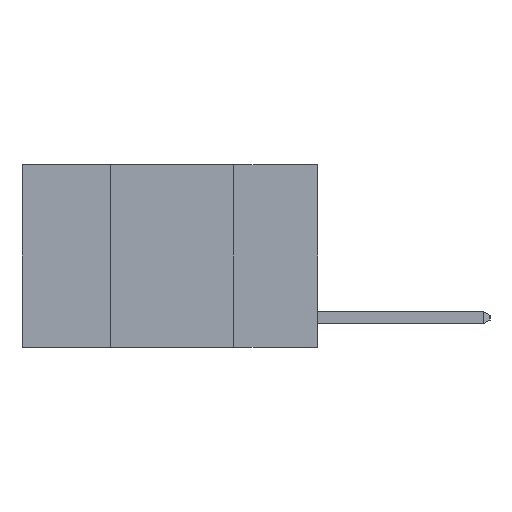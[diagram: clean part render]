
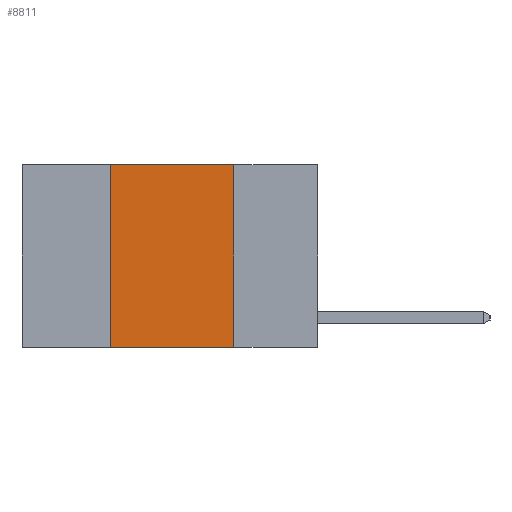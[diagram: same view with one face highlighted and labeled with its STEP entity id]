
A CAD part, left-side view. The second image highlights one B-rep face of the part: STEP entity #8811.
In plain terms, the highlighted planar face has unit normal (-1, 0, 0).
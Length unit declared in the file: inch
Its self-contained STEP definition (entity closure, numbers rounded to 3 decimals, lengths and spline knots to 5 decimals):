
#390 = ORIENTED_EDGE ( 'NONE', *, *, #4138, .F. ) ;
#1042 = VECTOR ( 'NONE', #3363, 39.37008 ) ;
#1397 = CARTESIAN_POINT ( 'NONE',  ( 0., 0.42, 0. ) ) ;
#1554 = LINE ( 'NONE', #7963, #3665 ) ;
#1672 = FACE_OUTER_BOUND ( 'NONE', #5782, .T. ) ;
#1971 = ORIENTED_EDGE ( 'NONE', *, *, #1982, .T. ) ;
#1982 = EDGE_CURVE ( 'NONE', #3238, #8017, #9057, .T. ) ;
#2132 = EDGE_CURVE ( 'NONE', #3238, #9530, #2167, .T. ) ;
#2167 = LINE ( 'NONE', #1397, #1042 ) ;
#2336 = EDGE_CURVE ( 'NONE', #4876, #8017, #5371, .T. ) ;
#2751 = VECTOR ( 'NONE', #6049, 39.37008 ) ;
#3035 = ORIENTED_EDGE ( 'NONE', *, *, #2336, .F. ) ;
#3158 = CARTESIAN_POINT ( 'NONE',  ( 0., 0.17, -0.37 ) ) ;
#3238 = VERTEX_POINT ( 'NONE', #9745 ) ;
#3363 = DIRECTION ( 'NONE',  ( 0., 0., 1. ) ) ;
#3376 = DIRECTION ( 'NONE',  ( 0., 0., -1. ) ) ;
#3378 = DIRECTION ( 'NONE',  ( 1., 0., 0. ) ) ;
#3538 = CARTESIAN_POINT ( 'NONE',  ( 0., 0.6, 0. ) ) ;
#3582 = PLANE ( 'NONE',  #5994 ) ;
#3665 = VECTOR ( 'NONE', #7187, 39.37008 ) ;
#4138 = EDGE_CURVE ( 'NONE', #9530, #4876, #1554, .T. ) ;
#4280 = CARTESIAN_POINT ( 'NONE',  ( 0., 0.17, 0. ) ) ;
#4876 = VERTEX_POINT ( 'NONE', #7511 ) ;
#5127 = CARTESIAN_POINT ( 'NONE',  ( 0., 0.42, 0. ) ) ;
#5371 = LINE ( 'NONE', #4280, #2751 ) ;
#5782 = EDGE_LOOP ( 'NONE', ( #3035, #390, #10269, #1971 ) ) ;
#5994 = AXIS2_PLACEMENT_3D ( 'NONE', #3538, #3378, #3376 ) ;
#6049 = DIRECTION ( 'NONE',  ( 0., 0., -1. ) ) ;
#7187 = DIRECTION ( 'NONE',  ( 0., -1., 0. ) ) ;
#7511 = CARTESIAN_POINT ( 'NONE',  ( 0., 0.17, 0. ) ) ;
#7963 = CARTESIAN_POINT ( 'NONE',  ( 0., 0.6, 0. ) ) ;
#8017 = VERTEX_POINT ( 'NONE', #3158 ) ;
#8135 = DIRECTION ( 'NONE',  ( 0., -1., 0. ) ) ;
#8811 = ADVANCED_FACE ( 'NONE', ( #1672 ), #3582, .F. ) ;
#8818 = VECTOR ( 'NONE', #8135, 39.37008 ) ;
#9057 = LINE ( 'NONE', #9456, #8818 ) ;
#9456 = CARTESIAN_POINT ( 'NONE',  ( 0., 0.6, -0.37 ) ) ;
#9530 = VERTEX_POINT ( 'NONE', #5127 ) ;
#9745 = CARTESIAN_POINT ( 'NONE',  ( 0., 0.42, -0.37 ) ) ;
#10269 = ORIENTED_EDGE ( 'NONE', *, *, #2132, .F. ) ;
